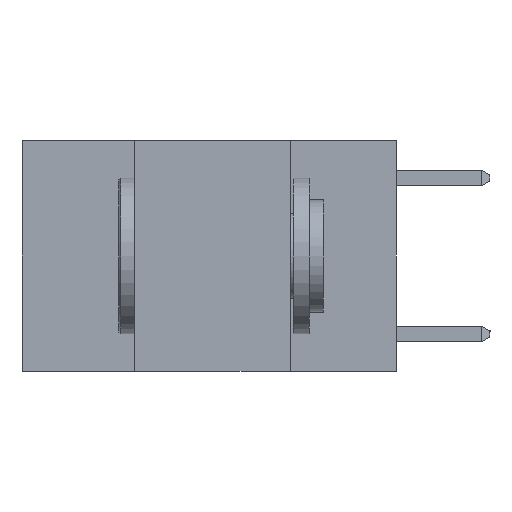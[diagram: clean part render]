
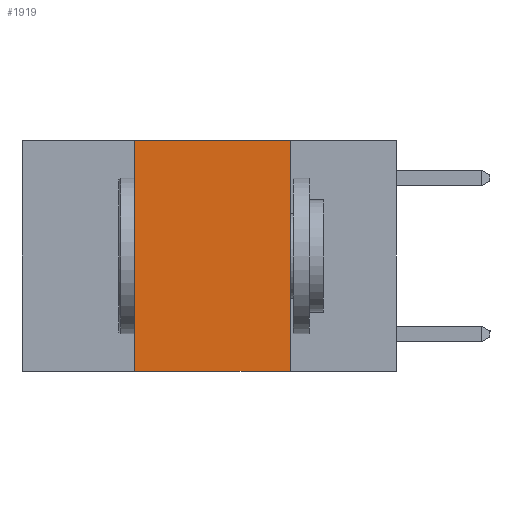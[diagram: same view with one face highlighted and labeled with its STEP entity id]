
A CAD part, left-side view. The second image highlights one B-rep face of the part: STEP entity #1919.
In plain terms, the highlighted planar face has unit normal (-1, 0, 0).
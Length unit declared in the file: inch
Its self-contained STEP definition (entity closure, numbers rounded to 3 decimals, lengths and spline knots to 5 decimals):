
#115 = LINE ( 'NONE', #1258, #5171 ) ;
#853 = LINE ( 'NONE', #3054, #10485 ) ;
#930 = DIRECTION ( 'NONE',  ( 0., 0., 1. ) ) ;
#1032 = VECTOR ( 'NONE', #1084, 39.37008 ) ;
#1038 = EDGE_CURVE ( 'NONE', #5134, #1523, #10836, .T. ) ;
#1084 = DIRECTION ( 'NONE',  ( 0., -1., 0. ) ) ;
#1258 = CARTESIAN_POINT ( 'NONE',  ( 0., 0.17, 0. ) ) ;
#1523 = VERTEX_POINT ( 'NONE', #1955 ) ;
#1680 = CARTESIAN_POINT ( 'NONE',  ( 0., 0.42, 0. ) ) ;
#1688 = VECTOR ( 'NONE', #6692, 39.37008 ) ;
#1919 = ADVANCED_FACE ( 'NONE', ( #3746 ), #7004, .F. ) ;
#1955 = CARTESIAN_POINT ( 'NONE',  ( 0., 0.17, 0. ) ) ;
#2252 = DIRECTION ( 'NONE',  ( 0., 0., -1. ) ) ;
#2317 = DIRECTION ( 'NONE',  ( 0., 0., -1. ) ) ;
#2562 = CARTESIAN_POINT ( 'NONE',  ( 0., 0.42, -0.37 ) ) ;
#3054 = CARTESIAN_POINT ( 'NONE',  ( 0., 0.42, 0. ) ) ;
#3087 = VERTEX_POINT ( 'NONE', #10554 ) ;
#3185 = CARTESIAN_POINT ( 'NONE',  ( 0., 0.6, -0.37 ) ) ;
#3383 = CARTESIAN_POINT ( 'NONE',  ( 0., 0.6, 0. ) ) ;
#3393 = AXIS2_PLACEMENT_3D ( 'NONE', #6955, #7910, #2252 ) ;
#3746 = FACE_OUTER_BOUND ( 'NONE', #11731, .T. ) ;
#3792 = LINE ( 'NONE', #3185, #1032 ) ;
#4553 = EDGE_CURVE ( 'NONE', #5890, #3087, #3792, .T. ) ;
#5134 = VERTEX_POINT ( 'NONE', #1680 ) ;
#5171 = VECTOR ( 'NONE', #2317, 39.37008 ) ;
#5396 = EDGE_CURVE ( 'NONE', #5890, #5134, #853, .T. ) ;
#5890 = VERTEX_POINT ( 'NONE', #2562 ) ;
#6692 = DIRECTION ( 'NONE',  ( 0., -1., 0. ) ) ;
#6955 = CARTESIAN_POINT ( 'NONE',  ( 0., 0.6, 0. ) ) ;
#7004 = PLANE ( 'NONE',  #3393 ) ;
#7279 = ORIENTED_EDGE ( 'NONE', *, *, #9667, .F. ) ;
#7465 = ORIENTED_EDGE ( 'NONE', *, *, #5396, .F. ) ;
#7910 = DIRECTION ( 'NONE',  ( 1., 0., 0. ) ) ;
#8109 = ORIENTED_EDGE ( 'NONE', *, *, #1038, .F. ) ;
#9571 = ORIENTED_EDGE ( 'NONE', *, *, #4553, .T. ) ;
#9667 = EDGE_CURVE ( 'NONE', #1523, #3087, #115, .T. ) ;
#10485 = VECTOR ( 'NONE', #930, 39.37008 ) ;
#10554 = CARTESIAN_POINT ( 'NONE',  ( 0., 0.17, -0.37 ) ) ;
#10836 = LINE ( 'NONE', #3383, #1688 ) ;
#11731 = EDGE_LOOP ( 'NONE', ( #7279, #8109, #7465, #9571 ) ) ;
